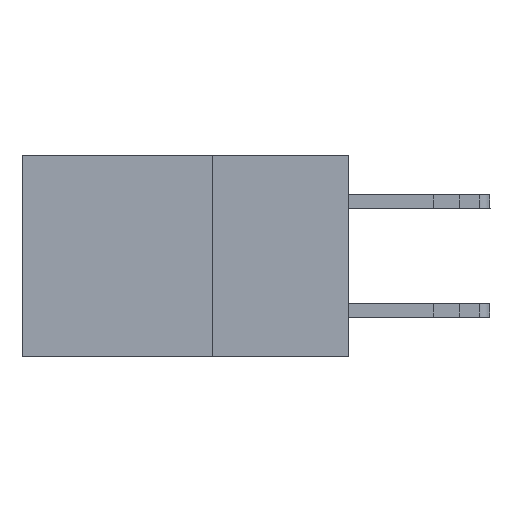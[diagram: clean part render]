
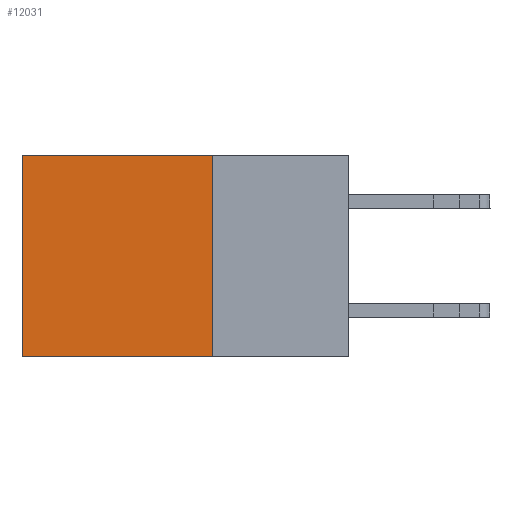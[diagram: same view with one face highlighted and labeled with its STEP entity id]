
A CAD part, left-side view. The second image highlights one B-rep face of the part: STEP entity #12031.
In plain terms, the highlighted planar face has unit normal (-1, 0, 0).
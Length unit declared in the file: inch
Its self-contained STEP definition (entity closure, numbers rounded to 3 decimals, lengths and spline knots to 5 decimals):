
#410 = DIRECTION ( 'NONE',  ( 0., 0., -1. ) ) ;
#803 = EDGE_CURVE ( 'NONE', #9121, #3687, #7101, .T. ) ;
#988 = DIRECTION ( 'NONE',  ( 0., 1., 0. ) ) ;
#1053 = ORIENTED_EDGE ( 'NONE', *, *, #6659, .T. ) ;
#1602 = VERTEX_POINT ( 'NONE', #10234 ) ;
#1917 = CARTESIAN_POINT ( 'NONE',  ( 0.2615, 0.25, -0.37 ) ) ;
#2263 = VECTOR ( 'NONE', #12155, 39.37008 ) ;
#2583 = CARTESIAN_POINT ( 'NONE',  ( 0.2615, 0.25, -0.37 ) ) ;
#3644 = AXIS2_PLACEMENT_3D ( 'NONE', #11072, #12289, #11325 ) ;
#3687 = VERTEX_POINT ( 'NONE', #1917 ) ;
#3688 = EDGE_CURVE ( 'NONE', #7398, #1602, #8682, .T. ) ;
#4493 = PLANE ( 'NONE',  #3644 ) ;
#6327 = ORIENTED_EDGE ( 'NONE', *, *, #803, .F. ) ;
#6397 = CARTESIAN_POINT ( 'NONE',  ( 0.2615, 0.6, 0. ) ) ;
#6659 = EDGE_CURVE ( 'NONE', #9121, #7398, #7766, .T. ) ;
#6939 = EDGE_CURVE ( 'NONE', #3687, #1602, #11256, .T. ) ;
#7101 = LINE ( 'NONE', #10983, #8662 ) ;
#7398 = VERTEX_POINT ( 'NONE', #6397 ) ;
#7716 = CARTESIAN_POINT ( 'NONE',  ( 0.2615, 0.25, 0. ) ) ;
#7766 = LINE ( 'NONE', #9801, #8978 ) ;
#8662 = VECTOR ( 'NONE', #410, 39.37008 ) ;
#8682 = LINE ( 'NONE', #11677, #11367 ) ;
#8978 = VECTOR ( 'NONE', #988, 39.37008 ) ;
#9121 = VERTEX_POINT ( 'NONE', #7716 ) ;
#9360 = FACE_OUTER_BOUND ( 'NONE', #9812, .T. ) ;
#9570 = ORIENTED_EDGE ( 'NONE', *, *, #6939, .F. ) ;
#9637 = ORIENTED_EDGE ( 'NONE', *, *, #3688, .T. ) ;
#9801 = CARTESIAN_POINT ( 'NONE',  ( 0.2615, 0.25, 0. ) ) ;
#9812 = EDGE_LOOP ( 'NONE', ( #9637, #9570, #6327, #1053 ) ) ;
#10234 = CARTESIAN_POINT ( 'NONE',  ( 0.2615, 0.6, -0.37 ) ) ;
#10780 = DIRECTION ( 'NONE',  ( 0., 0., -1. ) ) ;
#10983 = CARTESIAN_POINT ( 'NONE',  ( 0.2615, 0.25, -0.37 ) ) ;
#11072 = CARTESIAN_POINT ( 'NONE',  ( 0.2615, 0.25, -0.37 ) ) ;
#11256 = LINE ( 'NONE', #2583, #2263 ) ;
#11325 = DIRECTION ( 'NONE',  ( 0., 0., -1. ) ) ;
#11367 = VECTOR ( 'NONE', #10780, 39.37008 ) ;
#11677 = CARTESIAN_POINT ( 'NONE',  ( 0.2615, 0.6, -0.37 ) ) ;
#12031 = ADVANCED_FACE ( 'NONE', ( #9360 ), #4493, .F. ) ;
#12155 = DIRECTION ( 'NONE',  ( 0., 1., 0. ) ) ;
#12289 = DIRECTION ( 'NONE',  ( 1., 0., 0. ) ) ;
